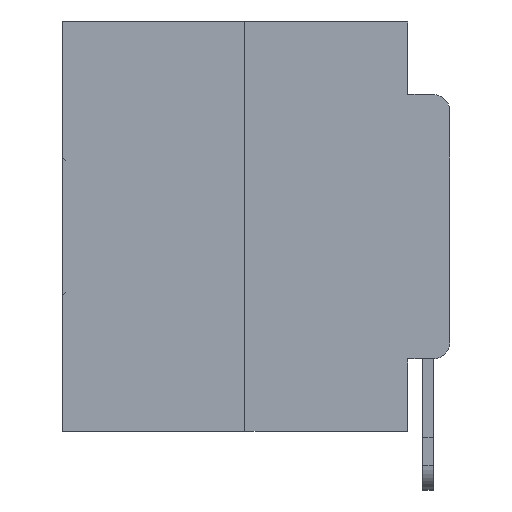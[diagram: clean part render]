
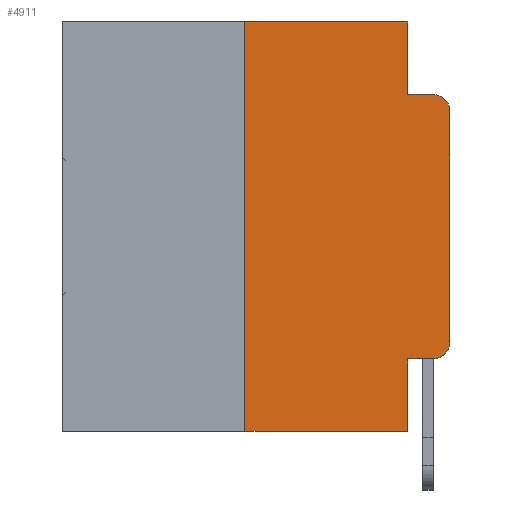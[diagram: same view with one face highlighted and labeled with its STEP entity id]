
A CAD part, left-side view. The second image highlights one B-rep face of the part: STEP entity #4911.
In plain terms, the highlighted planar face has unit normal (-1, 0, 0).
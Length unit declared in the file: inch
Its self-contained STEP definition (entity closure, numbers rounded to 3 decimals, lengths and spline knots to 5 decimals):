
#187 = EDGE_CURVE ( 'NONE', #31335, #6248, #18320, .T. ) ;
#1107 = CARTESIAN_POINT ( 'NONE',  ( 0., 0.473, 0. ) ) ;
#1505 = CARTESIAN_POINT ( 'NONE',  ( 0., 0.02, -0.0885 ) ) ;
#2495 = CARTESIAN_POINT ( 'NONE',  ( 0., 0.25, 0. ) ) ;
#2554 = CARTESIAN_POINT ( 'NONE',  ( 0., 0., -0.3915 ) ) ;
#2957 = CARTESIAN_POINT ( 'NONE',  ( 0., 0., -0.1085 ) ) ;
#3141 = EDGE_LOOP ( 'NONE', ( #21460, #11339, #21008, #27419, #4598, #18493, #21076, #21588, #22914, #23292 ) ) ;
#3571 = DIRECTION ( 'NONE',  ( 0., -1., 0. ) ) ;
#3657 = DIRECTION ( 'NONE',  ( 0., 0., -1. ) ) ;
#3761 = CARTESIAN_POINT ( 'NONE',  ( 0., 0.051, -0.0885 ) ) ;
#3803 = DIRECTION ( 'NONE',  ( 1., 0., 0. ) ) ;
#3808 = VECTOR ( 'NONE', #20739, 39.37008 ) ;
#3813 = VECTOR ( 'NONE', #3571, 39.37008 ) ;
#3830 = EDGE_CURVE ( 'NONE', #6413, #31335, #25013, .T. ) ;
#4532 = VECTOR ( 'NONE', #19291, 39.37008 ) ;
#4598 = ORIENTED_EDGE ( 'NONE', *, *, #13934, .F. ) ;
#4764 = VERTEX_POINT ( 'NONE', #15631 ) ;
#4911 = ADVANCED_FACE ( 'NONE', ( #10977 ), #16140, .F. ) ;
#5360 = VERTEX_POINT ( 'NONE', #2957 ) ;
#5531 = EDGE_CURVE ( 'NONE', #6413, #18608, #24088, .T. ) ;
#5736 = VERTEX_POINT ( 'NONE', #15274 ) ;
#6248 = VERTEX_POINT ( 'NONE', #2554 ) ;
#6413 = VERTEX_POINT ( 'NONE', #13165 ) ;
#6963 = CIRCLE ( 'NONE', #25170, 0.02 ) ;
#7232 = EDGE_CURVE ( 'NONE', #17534, #5736, #23977, .T. ) ;
#8935 = EDGE_CURVE ( 'NONE', #4764, #10927, #10910, .T. ) ;
#9760 = DIRECTION ( 'NONE',  ( 0., -1., 0. ) ) ;
#10592 = LINE ( 'NONE', #23054, #3808 ) ;
#10910 = LINE ( 'NONE', #13652, #27636 ) ;
#10927 = VERTEX_POINT ( 'NONE', #3761 ) ;
#10977 = FACE_OUTER_BOUND ( 'NONE', #3141, .T. ) ;
#11339 = ORIENTED_EDGE ( 'NONE', *, *, #15484, .T. ) ;
#11513 = EDGE_CURVE ( 'NONE', #17534, #18608, #10592, .T. ) ;
#11738 = VERTEX_POINT ( 'NONE', #1505 ) ;
#12313 = EDGE_CURVE ( 'NONE', #10927, #11738, #30202, .T. ) ;
#12487 = CARTESIAN_POINT ( 'NONE',  ( 0., 0.02, -0.1085 ) ) ;
#13165 = CARTESIAN_POINT ( 'NONE',  ( 0., 0.051, -0.4115 ) ) ;
#13652 = CARTESIAN_POINT ( 'NONE',  ( 0., 0.051, 0. ) ) ;
#13747 = DIRECTION ( 'NONE',  ( 0., -1., 0. ) ) ;
#13934 = EDGE_CURVE ( 'NONE', #5736, #4764, #18766, .T. ) ;
#14225 = LINE ( 'NONE', #21047, #26157 ) ;
#14858 = DIRECTION ( 'NONE',  ( 0., 0., -1. ) ) ;
#15274 = CARTESIAN_POINT ( 'NONE',  ( 0., 0.25, 0. ) ) ;
#15484 = EDGE_CURVE ( 'NONE', #5360, #11738, #6963, .T. ) ;
#15631 = CARTESIAN_POINT ( 'NONE',  ( 0., 0.051, 0. ) ) ;
#15928 = CARTESIAN_POINT ( 'NONE',  ( 0., 0.051, -0.0885 ) ) ;
#16140 = PLANE ( 'NONE',  #27441 ) ;
#17076 = EDGE_CURVE ( 'NONE', #6248, #5360, #14225, .T. ) ;
#17534 = VERTEX_POINT ( 'NONE', #30565 ) ;
#17538 = VECTOR ( 'NONE', #29212, 39.37008 ) ;
#18320 = CIRCLE ( 'NONE', #23657, 0.02 ) ;
#18493 = ORIENTED_EDGE ( 'NONE', *, *, #7232, .F. ) ;
#18608 = VERTEX_POINT ( 'NONE', #25230 ) ;
#18766 = LINE ( 'NONE', #30221, #30467 ) ;
#19291 = DIRECTION ( 'NONE',  ( 0., 0., -1. ) ) ;
#20739 = DIRECTION ( 'NONE',  ( 0., -1., 0. ) ) ;
#21003 = DIRECTION ( 'NONE',  ( 0., 0., -1. ) ) ;
#21008 = ORIENTED_EDGE ( 'NONE', *, *, #12313, .F. ) ;
#21047 = CARTESIAN_POINT ( 'NONE',  ( 0., 0., 0. ) ) ;
#21076 = ORIENTED_EDGE ( 'NONE', *, *, #11513, .T. ) ;
#21460 = ORIENTED_EDGE ( 'NONE', *, *, #17076, .T. ) ;
#21588 = ORIENTED_EDGE ( 'NONE', *, *, #5531, .F. ) ;
#22232 = DIRECTION ( 'NONE',  ( -1., 0., 0. ) ) ;
#22305 = CARTESIAN_POINT ( 'NONE',  ( 0., 0.02, -0.3915 ) ) ;
#22914 = ORIENTED_EDGE ( 'NONE', *, *, #3830, .T. ) ;
#23054 = CARTESIAN_POINT ( 'NONE',  ( 0., 0.473, -0.5 ) ) ;
#23292 = ORIENTED_EDGE ( 'NONE', *, *, #187, .T. ) ;
#23657 = AXIS2_PLACEMENT_3D ( 'NONE', #22305, #22232, #26329 ) ;
#23977 = LINE ( 'NONE', #2495, #17538 ) ;
#24088 = LINE ( 'NONE', #26424, #4532 ) ;
#24216 = CARTESIAN_POINT ( 'NONE',  ( 0., 0.051, -0.4115 ) ) ;
#25013 = LINE ( 'NONE', #24216, #30345 ) ;
#25170 = AXIS2_PLACEMENT_3D ( 'NONE', #12487, #28986, #14858 ) ;
#25230 = CARTESIAN_POINT ( 'NONE',  ( 0., 0.051, -0.5 ) ) ;
#26157 = VECTOR ( 'NONE', #28101, 39.37008 ) ;
#26329 = DIRECTION ( 'NONE',  ( 0., 0., -1. ) ) ;
#26424 = CARTESIAN_POINT ( 'NONE',  ( 0., 0.051, 0. ) ) ;
#27419 = ORIENTED_EDGE ( 'NONE', *, *, #8935, .F. ) ;
#27441 = AXIS2_PLACEMENT_3D ( 'NONE', #1107, #3803, #21003 ) ;
#27636 = VECTOR ( 'NONE', #3657, 39.37008 ) ;
#28101 = DIRECTION ( 'NONE',  ( 0., 0., 1. ) ) ;
#28986 = DIRECTION ( 'NONE',  ( -1., 0., 0. ) ) ;
#29212 = DIRECTION ( 'NONE',  ( 0., 0., 1. ) ) ;
#30202 = LINE ( 'NONE', #15928, #3813 ) ;
#30221 = CARTESIAN_POINT ( 'NONE',  ( 0., 0.473, 0. ) ) ;
#30345 = VECTOR ( 'NONE', #9760, 39.37008 ) ;
#30459 = CARTESIAN_POINT ( 'NONE',  ( 0., 0.02, -0.4115 ) ) ;
#30467 = VECTOR ( 'NONE', #13747, 39.37008 ) ;
#30565 = CARTESIAN_POINT ( 'NONE',  ( 0., 0.25, -0.5 ) ) ;
#31335 = VERTEX_POINT ( 'NONE', #30459 ) ;
